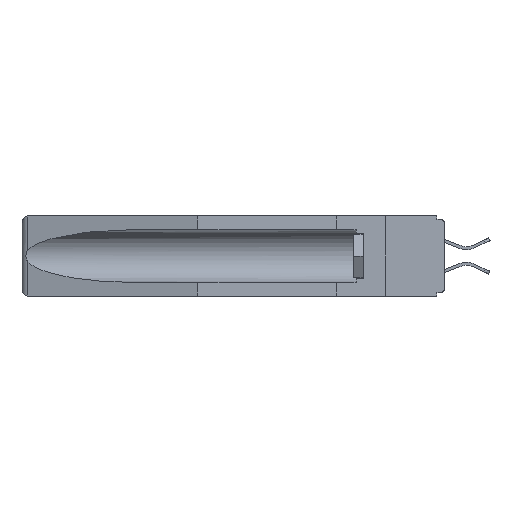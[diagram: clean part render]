
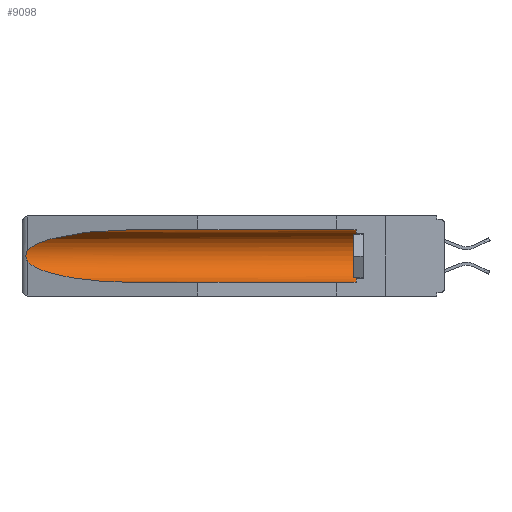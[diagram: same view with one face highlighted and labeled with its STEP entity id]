
A CAD part, left-side view. The second image highlights one B-rep face of the part: STEP entity #9098.
In plain terms, the highlighted cylindrical face has radius 2.857 mm (diameter 5.715 mm), a partial arc.
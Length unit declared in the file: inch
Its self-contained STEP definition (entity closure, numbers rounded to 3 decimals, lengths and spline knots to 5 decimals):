
#156 = DIRECTION ( 'NONE',  ( 0., 1., 0. ) ) ;
#408 = DIRECTION ( 'NONE',  ( 0., 0., 1. ) ) ;
#617 = LINE ( 'NONE', #9493, #3434 ) ;
#914 = ORIENTED_EDGE ( 'NONE', *, *, #8696, .T. ) ;
#1058 = DIRECTION ( 'NONE',  ( 0., 1., 0. ) ) ;
#1199 = CARTESIAN_POINT ( 'NONE',  ( 0.2673, 1.53269, -0.17917 ) ) ;
#1256 = VERTEX_POINT ( 'NONE', #18029 ) ;
#1408 = EDGE_LOOP ( 'NONE', ( #1696, #17087, #9888, #3588, #914, #13107 ) ) ;
#1457 = CARTESIAN_POINT ( 'NONE',  ( 0.26597, 1.5296, -0.19026 ) ) ;
#1696 = ORIENTED_EDGE ( 'NONE', *, *, #13151, .T. ) ;
#2540 = CARTESIAN_POINT ( 'NONE',  ( 0.26597, 1.52961, -0.15275 ) ) ;
#2690 = B_SPLINE_CURVE_WITH_KNOTS ( 'NONE', 3,
 ( #16703, #2540, #18351, #12536, #11227, #12666, #1199, #4074, #1457, #14142 ),
 .UNSPECIFIED., .F., .F.,
 ( 4, 2, 2, 2, 4 ),
 ( 0., 0.00029, 0.00058, 0.00087, 0.00117 ),
 .UNSPECIFIED. ) ;
#3090 = CARTESIAN_POINT ( 'NONE',  ( 0.26537, 1.52718, -0.19328 ) ) ;
#3137 = CARTESIAN_POINT ( 'NONE',  ( 0.155, 0.126, -0.059 ) ) ;
#3434 = VECTOR ( 'NONE', #1058, 39.37008 ) ;
#3471 = CARTESIAN_POINT ( 'NONE',  ( 0.155, -0.30754, -0.059 ) ) ;
#3588 = ORIENTED_EDGE ( 'NONE', *, *, #7473, .F. ) ;
#4036 =( BOUNDED_CURVE ( )  B_SPLINE_CURVE ( 3, ( #10923, #12417, #13734, #15320 ),
 .UNSPECIFIED., .F., .F. ) 
 B_SPLINE_CURVE_WITH_KNOTS ( ( 4, 4 ),
 ( 4.71239, 6.08839 ),
 .UNSPECIFIED. ) 
 CURVE ( )  GEOMETRIC_REPRESENTATION_ITEM ( )  RATIONAL_B_SPLINE_CURVE ( ( 1., 0.848, 0.848, 1. ) ) 
 REPRESENTATION_ITEM ( '' )  );
#4074 = CARTESIAN_POINT ( 'NONE',  ( 0.26655, 1.53094, -0.18657 ) ) ;
#4323 = CARTESIAN_POINT ( 'NONE',  ( 0.155, 1.07973, -0.284 ) ) ;
#4438 = VERTEX_POINT ( 'NONE', #8135 ) ;
#5472 = AXIS2_PLACEMENT_3D ( 'NONE', #9155, #156, #13991 ) ;
#5568 = LINE ( 'NONE', #3471, #9123 ) ;
#5661 = VERTEX_POINT ( 'NONE', #3137 ) ;
#5689 = CARTESIAN_POINT ( 'NONE',  ( 0.25451, 1.48313, -0.24835 ) ) ;
#6447 = EDGE_CURVE ( 'NONE', #14000, #1256, #6758, .T. ) ;
#6670 = CARTESIAN_POINT ( 'NONE',  ( 0.155, 0.126, -0.284 ) ) ;
#6758 =( BOUNDED_CURVE ( )  B_SPLINE_CURVE ( 3, ( #3090, #5689, #17268, #4323 ),
 .UNSPECIFIED., .F., .F. ) 
 B_SPLINE_CURVE_WITH_KNOTS ( ( 4, 4 ),
 ( 0.1948, 1.5708 ),
 .UNSPECIFIED. ) 
 CURVE ( )  GEOMETRIC_REPRESENTATION_ITEM ( )  RATIONAL_B_SPLINE_CURVE ( ( 1., 0.848, 0.848, 1. ) ) 
 REPRESENTATION_ITEM ( '' )  );
#7223 = AXIS2_PLACEMENT_3D ( 'NONE', #11852, #7398, #408 ) ;
#7398 = DIRECTION ( 'NONE',  ( 0., -1., 0. ) ) ;
#7473 = EDGE_CURVE ( 'NONE', #15467, #1256, #617, .T. ) ;
#7693 = CARTESIAN_POINT ( 'NONE',  ( 0.26537, 1.52718, -0.14972 ) ) ;
#7707 = FACE_OUTER_BOUND ( 'NONE', #1408, .T. ) ;
#7725 = CIRCLE ( 'NONE', #7223, 0.1125 ) ;
#7877 = EDGE_CURVE ( 'NONE', #18134, #14000, #2690, .T. ) ;
#7930 = CYLINDRICAL_SURFACE ( 'NONE', #5472, 0.1125 ) ;
#8135 = CARTESIAN_POINT ( 'NONE',  ( 0.155, 1.07973, -0.059 ) ) ;
#8696 = EDGE_CURVE ( 'NONE', #15467, #5661, #7725, .T. ) ;
#9098 = ADVANCED_FACE ( 'NONE', ( #7707 ), #7930, .F. ) ;
#9123 = VECTOR ( 'NONE', #13423, 39.37008 ) ;
#9155 = CARTESIAN_POINT ( 'NONE',  ( 0.155, -0.30754, -0.1715 ) ) ;
#9493 = CARTESIAN_POINT ( 'NONE',  ( 0.155, -0.30754, -0.284 ) ) ;
#9888 = ORIENTED_EDGE ( 'NONE', *, *, #6447, .T. ) ;
#10923 = CARTESIAN_POINT ( 'NONE',  ( 0.155, 1.07973, -0.059 ) ) ;
#10955 = CARTESIAN_POINT ( 'NONE',  ( 0.26537, 1.52718, -0.19328 ) ) ;
#11227 = CARTESIAN_POINT ( 'NONE',  ( 0.2675, 1.53308, -0.16763 ) ) ;
#11852 = CARTESIAN_POINT ( 'NONE',  ( 0.155, 0.126, -0.1715 ) ) ;
#12417 = CARTESIAN_POINT ( 'NONE',  ( 0.21114, 1.30732, -0.059 ) ) ;
#12536 = CARTESIAN_POINT ( 'NONE',  ( 0.2673, 1.5327, -0.16383 ) ) ;
#12666 = CARTESIAN_POINT ( 'NONE',  ( 0.2675, 1.53308, -0.17534 ) ) ;
#13107 = ORIENTED_EDGE ( 'NONE', *, *, #15272, .T. ) ;
#13151 = EDGE_CURVE ( 'NONE', #4438, #18134, #4036, .T. ) ;
#13423 = DIRECTION ( 'NONE',  ( 0., 1., 0. ) ) ;
#13734 = CARTESIAN_POINT ( 'NONE',  ( 0.25451, 1.48313, -0.09465 ) ) ;
#13991 = DIRECTION ( 'NONE',  ( 0., 0., 1. ) ) ;
#14000 = VERTEX_POINT ( 'NONE', #10955 ) ;
#14142 = CARTESIAN_POINT ( 'NONE',  ( 0.26537, 1.52718, -0.19328 ) ) ;
#15272 = EDGE_CURVE ( 'NONE', #5661, #4438, #5568, .T. ) ;
#15320 = CARTESIAN_POINT ( 'NONE',  ( 0.26537, 1.52718, -0.14972 ) ) ;
#15467 = VERTEX_POINT ( 'NONE', #6670 ) ;
#16703 = CARTESIAN_POINT ( 'NONE',  ( 0.26537, 1.52718, -0.14972 ) ) ;
#17087 = ORIENTED_EDGE ( 'NONE', *, *, #7877, .T. ) ;
#17268 = CARTESIAN_POINT ( 'NONE',  ( 0.21114, 1.30732, -0.284 ) ) ;
#18029 = CARTESIAN_POINT ( 'NONE',  ( 0.155, 1.07973, -0.284 ) ) ;
#18134 = VERTEX_POINT ( 'NONE', #7693 ) ;
#18351 = CARTESIAN_POINT ( 'NONE',  ( 0.26654, 1.53092, -0.15636 ) ) ;
